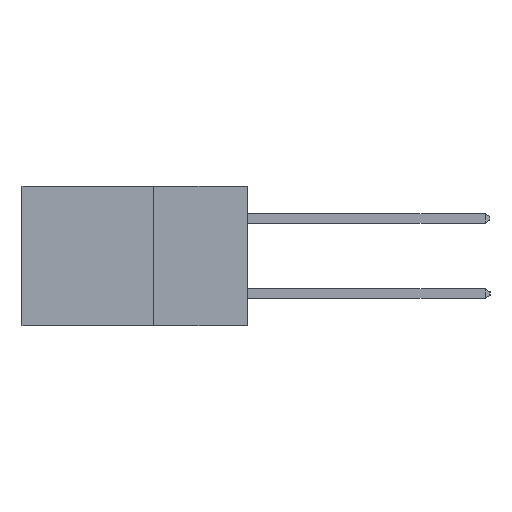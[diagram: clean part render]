
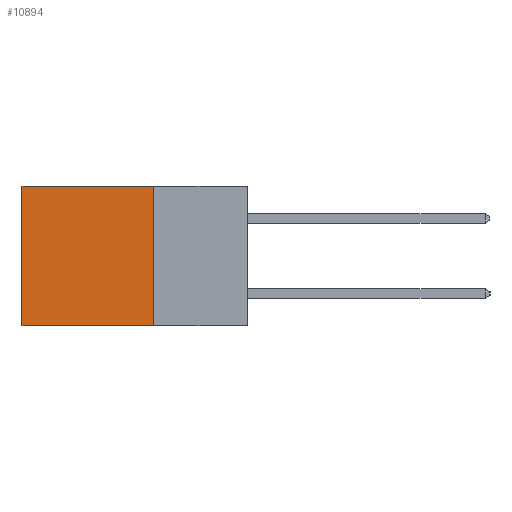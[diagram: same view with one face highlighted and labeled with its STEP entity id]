
A CAD part, left-side view. The second image highlights one B-rep face of the part: STEP entity #10894.
In plain terms, the highlighted planar face has unit normal (-1, 0, 0).
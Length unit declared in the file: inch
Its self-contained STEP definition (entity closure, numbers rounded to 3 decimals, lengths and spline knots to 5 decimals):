
#143 = DIRECTION ( 'NONE',  ( 0., 0., -1. ) ) ;
#180 = EDGE_CURVE ( 'NONE', #15929, #9699, #21436, .T. ) ;
#1323 = ORIENTED_EDGE ( 'NONE', *, *, #180, .T. ) ;
#1542 = PLANE ( 'NONE',  #18267 ) ;
#1896 = EDGE_CURVE ( 'NONE', #21904, #9699, #12715, .T. ) ;
#2439 = CARTESIAN_POINT ( 'NONE',  ( 0.2615, 0.25, 0. ) ) ;
#5333 = EDGE_CURVE ( 'NONE', #14103, #21904, #23933, .T. ) ;
#5555 = DIRECTION ( 'NONE',  ( 1., 0., 0. ) ) ;
#5968 = CARTESIAN_POINT ( 'NONE',  ( 0.2615, 0.6, 0. ) ) ;
#6631 = FACE_OUTER_BOUND ( 'NONE', #25508, .T. ) ;
#6830 = DIRECTION ( 'NONE',  ( 0., 1., 0. ) ) ;
#7886 = CARTESIAN_POINT ( 'NONE',  ( 0.2615, 0.25, -0.37 ) ) ;
#8362 = EDGE_CURVE ( 'NONE', #14103, #15929, #18016, .T. ) ;
#8528 = CARTESIAN_POINT ( 'NONE',  ( 0.2615, 0.25, -0.37 ) ) ;
#8560 = CARTESIAN_POINT ( 'NONE',  ( 0.2615, 0.6, -0.37 ) ) ;
#9699 = VERTEX_POINT ( 'NONE', #10283 ) ;
#10283 = CARTESIAN_POINT ( 'NONE',  ( 0.2615, 0.6, -0.37 ) ) ;
#10894 = ADVANCED_FACE ( 'NONE', ( #6631 ), #1542, .F. ) ;
#10914 = VECTOR ( 'NONE', #11416, 39.37008 ) ;
#11416 = DIRECTION ( 'NONE',  ( 0., 0., -1. ) ) ;
#11773 = ORIENTED_EDGE ( 'NONE', *, *, #8362, .T. ) ;
#12715 = LINE ( 'NONE', #8528, #21951 ) ;
#12754 = VECTOR ( 'NONE', #20406, 39.37008 ) ;
#14103 = VERTEX_POINT ( 'NONE', #17848 ) ;
#15929 = VERTEX_POINT ( 'NONE', #5968 ) ;
#17566 = CARTESIAN_POINT ( 'NONE',  ( 0.2615, 0.25, -0.37 ) ) ;
#17848 = CARTESIAN_POINT ( 'NONE',  ( 0.2615, 0.25, 0. ) ) ;
#17939 = ORIENTED_EDGE ( 'NONE', *, *, #5333, .F. ) ;
#18016 = LINE ( 'NONE', #2439, #12754 ) ;
#18267 = AXIS2_PLACEMENT_3D ( 'NONE', #17566, #5555, #19520 ) ;
#18761 = VECTOR ( 'NONE', #143, 39.37008 ) ;
#19520 = DIRECTION ( 'NONE',  ( 0., 0., -1. ) ) ;
#20406 = DIRECTION ( 'NONE',  ( 0., 1., 0. ) ) ;
#21237 = ORIENTED_EDGE ( 'NONE', *, *, #1896, .F. ) ;
#21436 = LINE ( 'NONE', #8560, #10914 ) ;
#21904 = VERTEX_POINT ( 'NONE', #7886 ) ;
#21951 = VECTOR ( 'NONE', #6830, 39.37008 ) ;
#23927 = CARTESIAN_POINT ( 'NONE',  ( 0.2615, 0.25, -0.37 ) ) ;
#23933 = LINE ( 'NONE', #23927, #18761 ) ;
#25508 = EDGE_LOOP ( 'NONE', ( #1323, #21237, #17939, #11773 ) ) ;
